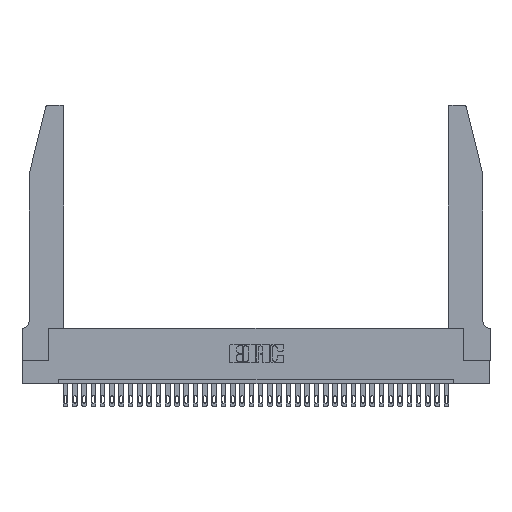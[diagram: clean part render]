
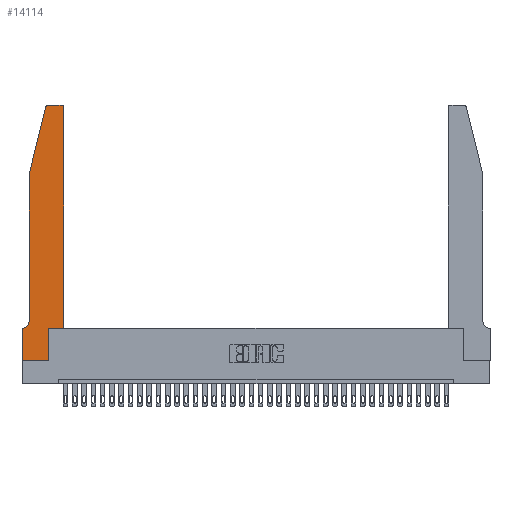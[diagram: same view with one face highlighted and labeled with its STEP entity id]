
A CAD part, top view. The second image highlights one B-rep face of the part: STEP entity #14114.
In plain terms, the highlighted planar face has unit normal (0, 0, 1).
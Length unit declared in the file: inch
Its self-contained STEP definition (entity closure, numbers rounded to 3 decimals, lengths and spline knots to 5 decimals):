
#394 = ORIENTED_EDGE ( 'NONE', *, *, #2692, .T. ) ;
#659 = VERTEX_POINT ( 'NONE', #5645 ) ;
#782 = DIRECTION ( 'NONE',  ( 0., 0., 1. ) ) ;
#1392 = DIRECTION ( 'NONE',  ( -1., 0., 0. ) ) ;
#1415 = DIRECTION ( 'NONE',  ( 1., 0., 0. ) ) ;
#2311 = LINE ( 'NONE', #25547, #6213 ) ;
#2383 = CARTESIAN_POINT ( 'NONE',  ( 0.0755, 2., 0.37 ) ) ;
#2692 = EDGE_CURVE ( 'NONE', #21695, #32723, #28507, .T. ) ;
#2959 = CARTESIAN_POINT ( 'NONE',  ( 0., 0.35, 0.37 ) ) ;
#3004 = AXIS2_PLACEMENT_3D ( 'NONE', #2959, #25140, #7954 ) ;
#3732 = EDGE_LOOP ( 'NONE', ( #12549, #29292, #394, #28130, #4335, #18259, #11284, #30098, #19948, #22667, #29941, #21237 ) ) ;
#4180 = VECTOR ( 'NONE', #8384, 39.37008 ) ;
#4328 = CARTESIAN_POINT ( 'NONE',  ( 0.2865, 0.35, 0.37 ) ) ;
#4335 = ORIENTED_EDGE ( 'NONE', *, *, #25901, .T. ) ;
#5380 = CARTESIAN_POINT ( 'NONE',  ( 0.284, 2.72, 0.37 ) ) ;
#5645 = CARTESIAN_POINT ( 'NONE',  ( 0.4505, 2.72, 0.37 ) ) ;
#5925 = LINE ( 'NONE', #16709, #4180 ) ;
#6025 = DIRECTION ( 'NONE',  ( 1., 0., 0. ) ) ;
#6213 = VECTOR ( 'NONE', #9089, 39.37008 ) ;
#6345 = CARTESIAN_POINT ( 'NONE',  ( 0.2865, 0.35, 0.37 ) ) ;
#6569 = EDGE_CURVE ( 'NONE', #19825, #659, #14547, .T. ) ;
#7954 = DIRECTION ( 'NONE',  ( 1., 0., 0. ) ) ;
#8037 = DIRECTION ( 'NONE',  ( 1., 0., 0. ) ) ;
#8111 = VECTOR ( 'NONE', #29087, 39.37008 ) ;
#8384 = DIRECTION ( 'NONE',  ( 0., -1., 0. ) ) ;
#8850 = CARTESIAN_POINT ( 'NONE',  ( 0.0055, 0.35, 0.37 ) ) ;
#9089 = DIRECTION ( 'NONE',  ( 0., -1., 0. ) ) ;
#10179 = CARTESIAN_POINT ( 'NONE',  ( 0.0055, 0.42, 0.37 ) ) ;
#10745 = VERTEX_POINT ( 'NONE', #34453 ) ;
#11284 = ORIENTED_EDGE ( 'NONE', *, *, #16218, .T. ) ;
#11629 = CARTESIAN_POINT ( 'NONE',  ( 0.4205, 2.72, 0.37 ) ) ;
#11674 = EDGE_CURVE ( 'NONE', #32723, #12703, #2311, .T. ) ;
#11750 = VECTOR ( 'NONE', #6025, 39.37008 ) ;
#12549 = ORIENTED_EDGE ( 'NONE', *, *, #27566, .T. ) ;
#12703 = VERTEX_POINT ( 'NONE', #20797 ) ;
#13567 = VERTEX_POINT ( 'NONE', #23935 ) ;
#14114 = ADVANCED_FACE ( 'NONE', ( #15255 ), #19686, .T. ) ;
#14547 = LINE ( 'NONE', #31651, #16760 ) ;
#14848 = VECTOR ( 'NONE', #19991, 39.37008 ) ;
#15255 = FACE_OUTER_BOUND ( 'NONE', #3732, .T. ) ;
#15548 = VECTOR ( 'NONE', #1415, 39.37008 ) ;
#15730 = AXIS2_PLACEMENT_3D ( 'NONE', #10179, #32635, #35553 ) ;
#15869 = CARTESIAN_POINT ( 'NONE',  ( 0.25487, 2.72718, 0.37 ) ) ;
#16218 = EDGE_CURVE ( 'NONE', #10745, #32601, #5925, .T. ) ;
#16335 = VERTEX_POINT ( 'NONE', #8850 ) ;
#16709 = CARTESIAN_POINT ( 'NONE',  ( 0., 0., 0.37 ) ) ;
#16760 = VECTOR ( 'NONE', #32142, 39.37008 ) ;
#16846 = DIRECTION ( 'NONE',  ( 0., 0., 1. ) ) ;
#17146 = EDGE_CURVE ( 'NONE', #16335, #10745, #31261, .T. ) ;
#18259 = ORIENTED_EDGE ( 'NONE', *, *, #17146, .T. ) ;
#19589 = CARTESIAN_POINT ( 'NONE',  ( 0.4505, 0.35, 0.37 ) ) ;
#19623 = LINE ( 'NONE', #19589, #11750 ) ;
#19686 = PLANE ( 'NONE',  #3004 ) ;
#19749 = CARTESIAN_POINT ( 'NONE',  ( 0.0755, 2., 0.37 ) ) ;
#19825 = VERTEX_POINT ( 'NONE', #21643 ) ;
#19915 = EDGE_CURVE ( 'NONE', #35285, #21695, #20552, .T. ) ;
#19948 = ORIENTED_EDGE ( 'NONE', *, *, #31559, .T. ) ;
#19991 = DIRECTION ( 'NONE',  ( -0.239, -0.971, 0. ) ) ;
#20071 = DIRECTION ( 'NONE',  ( 1., 0., 0. ) ) ;
#20552 = CIRCLE ( 'NONE', #24538, 0.03 ) ;
#20797 = CARTESIAN_POINT ( 'NONE',  ( 0.0755, 0.42, 0.37 ) ) ;
#21237 = ORIENTED_EDGE ( 'NONE', *, *, #28173, .T. ) ;
#21643 = CARTESIAN_POINT ( 'NONE',  ( 0.4505, 0.35, 0.37 ) ) ;
#21695 = VERTEX_POINT ( 'NONE', #15869 ) ;
#21765 = VECTOR ( 'NONE', #23742, 39.37008 ) ;
#22613 = LINE ( 'NONE', #6345, #21765 ) ;
#22667 = ORIENTED_EDGE ( 'NONE', *, *, #29810, .T. ) ;
#23084 = CARTESIAN_POINT ( 'NONE',  ( 0., 0., 0.37 ) ) ;
#23446 = CIRCLE ( 'NONE', #34613, 0.03 ) ;
#23448 = CARTESIAN_POINT ( 'NONE',  ( 0.2605, 2.75, 0.37 ) ) ;
#23742 = DIRECTION ( 'NONE',  ( 0., 1., 0. ) ) ;
#23935 = CARTESIAN_POINT ( 'NONE',  ( 0.4205, 2.75, 0.37 ) ) ;
#24538 = AXIS2_PLACEMENT_3D ( 'NONE', #5380, #16846, #8037 ) ;
#25140 = DIRECTION ( 'NONE',  ( 0., 0., 1. ) ) ;
#25547 = CARTESIAN_POINT ( 'NONE',  ( 0.0755, 2., 0.37 ) ) ;
#25901 = EDGE_CURVE ( 'NONE', #12703, #16335, #28002, .T. ) ;
#26670 = VERTEX_POINT ( 'NONE', #36123 ) ;
#27566 = EDGE_CURVE ( 'NONE', #13567, #35285, #28748, .T. ) ;
#28002 = CIRCLE ( 'NONE', #15730, 0.07 ) ;
#28130 = ORIENTED_EDGE ( 'NONE', *, *, #11674, .T. ) ;
#28173 = EDGE_CURVE ( 'NONE', #659, #13567, #23446, .T. ) ;
#28507 = LINE ( 'NONE', #19749, #14848 ) ;
#28748 = LINE ( 'NONE', #23448, #8111 ) ;
#29087 = DIRECTION ( 'NONE',  ( -1., 0., 0. ) ) ;
#29292 = ORIENTED_EDGE ( 'NONE', *, *, #19915, .T. ) ;
#29555 = CARTESIAN_POINT ( 'NONE',  ( 0.0755, 0.35, 0.37 ) ) ;
#29810 = EDGE_CURVE ( 'NONE', #35369, #19825, #19623, .T. ) ;
#29941 = ORIENTED_EDGE ( 'NONE', *, *, #6569, .T. ) ;
#30098 = ORIENTED_EDGE ( 'NONE', *, *, #32303, .T. ) ;
#30518 = LINE ( 'NONE', #23084, #15548 ) ;
#31261 = LINE ( 'NONE', #29555, #34296 ) ;
#31559 = EDGE_CURVE ( 'NONE', #26670, #35369, #22613, .T. ) ;
#31651 = CARTESIAN_POINT ( 'NONE',  ( 0.4505, 0.35, 0.37 ) ) ;
#32142 = DIRECTION ( 'NONE',  ( 0., 1., 0. ) ) ;
#32303 = EDGE_CURVE ( 'NONE', #32601, #26670, #30518, .T. ) ;
#32601 = VERTEX_POINT ( 'NONE', #35811 ) ;
#32635 = DIRECTION ( 'NONE',  ( 0., 0., -1. ) ) ;
#32723 = VERTEX_POINT ( 'NONE', #2383 ) ;
#34182 = CARTESIAN_POINT ( 'NONE',  ( 0.284, 2.75, 0.37 ) ) ;
#34296 = VECTOR ( 'NONE', #1392, 39.37008 ) ;
#34453 = CARTESIAN_POINT ( 'NONE',  ( 0., 0.35, 0.37 ) ) ;
#34613 = AXIS2_PLACEMENT_3D ( 'NONE', #11629, #782, #20071 ) ;
#35285 = VERTEX_POINT ( 'NONE', #34182 ) ;
#35369 = VERTEX_POINT ( 'NONE', #4328 ) ;
#35553 = DIRECTION ( 'NONE',  ( -1., 0., 0. ) ) ;
#35811 = CARTESIAN_POINT ( 'NONE',  ( 0., 0., 0.37 ) ) ;
#36123 = CARTESIAN_POINT ( 'NONE',  ( 0.2865, 0., 0.37 ) ) ;
